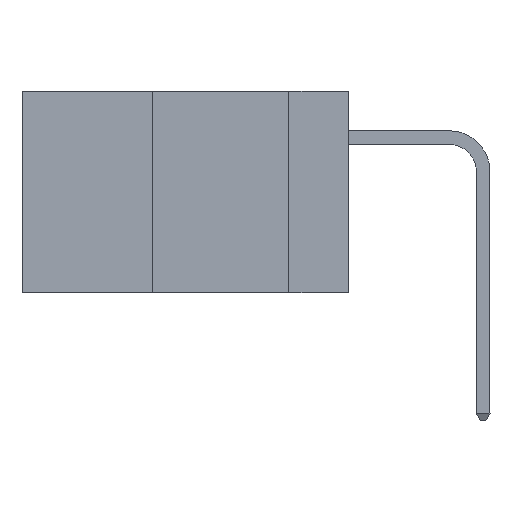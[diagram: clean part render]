
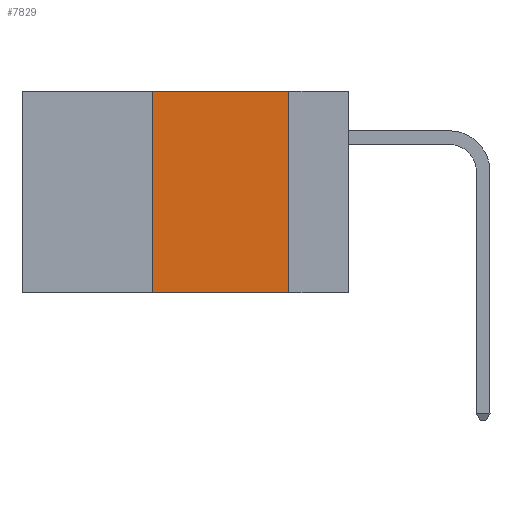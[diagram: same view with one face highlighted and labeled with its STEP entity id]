
A CAD part, left-side view. The second image highlights one B-rep face of the part: STEP entity #7829.
In plain terms, the highlighted planar face has unit normal (-1, 0, 0).
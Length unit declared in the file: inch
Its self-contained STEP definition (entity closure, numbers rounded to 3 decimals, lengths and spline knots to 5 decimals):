
#873 = CARTESIAN_POINT ( 'NONE',  ( 0., 0.11, 0. ) ) ;
#903 = PLANE ( 'NONE',  #1472 ) ;
#1127 = EDGE_CURVE ( 'NONE', #14273, #17291, #10315, .T. ) ;
#1282 = LINE ( 'NONE', #5337, #1802 ) ;
#1381 = LINE ( 'NONE', #5609, #16217 ) ;
#1472 = AXIS2_PLACEMENT_3D ( 'NONE', #17035, #4955, #2550 ) ;
#1544 = CARTESIAN_POINT ( 'NONE',  ( 0., 0.6, -0.37 ) ) ;
#1802 = VECTOR ( 'NONE', #13432, 39.37008 ) ;
#2436 = VERTEX_POINT ( 'NONE', #15874 ) ;
#2550 = DIRECTION ( 'NONE',  ( 0., 0., -1. ) ) ;
#4955 = DIRECTION ( 'NONE',  ( 1., 0., 0. ) ) ;
#5337 = CARTESIAN_POINT ( 'NONE',  ( 0., 0.6, 0. ) ) ;
#5447 = EDGE_CURVE ( 'NONE', #16236, #2436, #1381, .T. ) ;
#5609 = CARTESIAN_POINT ( 'NONE',  ( 0., 0.36, 0. ) ) ;
#5905 = CARTESIAN_POINT ( 'NONE',  ( 0., 0.11, -0.37 ) ) ;
#6245 = DIRECTION ( 'NONE',  ( 0., 0., -1. ) ) ;
#6839 = DIRECTION ( 'NONE',  ( 0., 0., 1. ) ) ;
#7322 = CARTESIAN_POINT ( 'NONE',  ( 0., 0.11, 0. ) ) ;
#7589 = FACE_OUTER_BOUND ( 'NONE', #13265, .T. ) ;
#7829 = ADVANCED_FACE ( 'NONE', ( #7589 ), #903, .F. ) ;
#9796 = VECTOR ( 'NONE', #14598, 39.37008 ) ;
#9968 = ORIENTED_EDGE ( 'NONE', *, *, #16127, .T. ) ;
#10315 = LINE ( 'NONE', #873, #14499 ) ;
#11072 = CARTESIAN_POINT ( 'NONE',  ( 0., 0.36, -0.37 ) ) ;
#12259 = EDGE_CURVE ( 'NONE', #2436, #14273, #1282, .T. ) ;
#13265 = EDGE_LOOP ( 'NONE', ( #14674, #15207, #15244, #9968 ) ) ;
#13432 = DIRECTION ( 'NONE',  ( 0., -1., 0. ) ) ;
#14273 = VERTEX_POINT ( 'NONE', #7322 ) ;
#14499 = VECTOR ( 'NONE', #6245, 39.37008 ) ;
#14598 = DIRECTION ( 'NONE',  ( 0., -1., 0. ) ) ;
#14674 = ORIENTED_EDGE ( 'NONE', *, *, #1127, .F. ) ;
#14685 = LINE ( 'NONE', #1544, #9796 ) ;
#15207 = ORIENTED_EDGE ( 'NONE', *, *, #12259, .F. ) ;
#15244 = ORIENTED_EDGE ( 'NONE', *, *, #5447, .F. ) ;
#15874 = CARTESIAN_POINT ( 'NONE',  ( 0., 0.36, 0. ) ) ;
#16127 = EDGE_CURVE ( 'NONE', #16236, #17291, #14685, .T. ) ;
#16217 = VECTOR ( 'NONE', #6839, 39.37008 ) ;
#16236 = VERTEX_POINT ( 'NONE', #11072 ) ;
#17035 = CARTESIAN_POINT ( 'NONE',  ( 0., 0.6, 0. ) ) ;
#17291 = VERTEX_POINT ( 'NONE', #5905 ) ;
